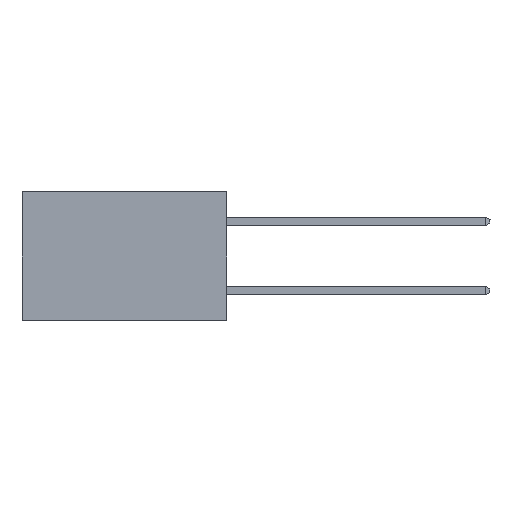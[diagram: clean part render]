
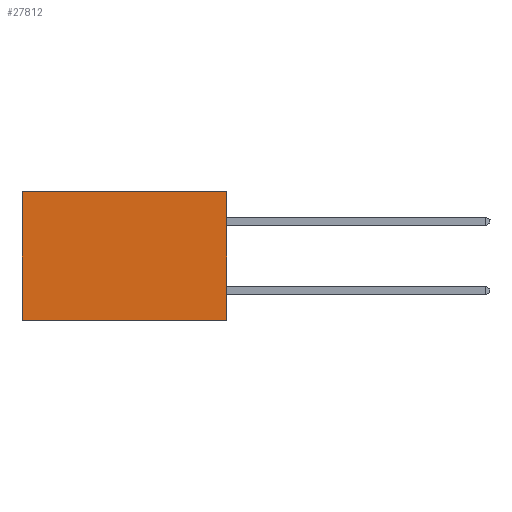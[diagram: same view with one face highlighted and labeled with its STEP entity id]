
A CAD part, left-side view. The second image highlights one B-rep face of the part: STEP entity #27812.
In plain terms, the highlighted planar face has unit normal (-1, 0, 0).
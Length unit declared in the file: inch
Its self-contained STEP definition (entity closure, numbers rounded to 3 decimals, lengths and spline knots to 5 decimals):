
#1165 = CARTESIAN_POINT ( 'NONE',  ( 0.277, 0.59, -0.37 ) ) ;
#3208 = LINE ( 'NONE', #18784, #22879 ) ;
#3996 = DIRECTION ( 'NONE',  ( 0., 0., -1. ) ) ;
#4317 = VECTOR ( 'NONE', #29599, 39.37008 ) ;
#4749 = LINE ( 'NONE', #11071, #30061 ) ;
#8733 = ORIENTED_EDGE ( 'NONE', *, *, #12134, .F. ) ;
#9128 = VERTEX_POINT ( 'NONE', #13149 ) ;
#10547 = VERTEX_POINT ( 'NONE', #1165 ) ;
#11071 = CARTESIAN_POINT ( 'NONE',  ( 0.277, 0., 0. ) ) ;
#12134 = EDGE_CURVE ( 'NONE', #9128, #20420, #3208, .T. ) ;
#12529 = CARTESIAN_POINT ( 'NONE',  ( 0.277, 0.59, -0.37 ) ) ;
#13149 = CARTESIAN_POINT ( 'NONE',  ( 0.277, 0., 0. ) ) ;
#13502 = DIRECTION ( 'NONE',  ( 0., 1., 0. ) ) ;
#13918 = EDGE_CURVE ( 'NONE', #24196, #10547, #23184, .T. ) ;
#14272 = PLANE ( 'NONE',  #29160 ) ;
#14430 = ORIENTED_EDGE ( 'NONE', *, *, #13918, .T. ) ;
#15131 = EDGE_LOOP ( 'NONE', ( #14430, #27126, #8733, #29062 ) ) ;
#16356 = CARTESIAN_POINT ( 'NONE',  ( 0.277, 0.59, 0. ) ) ;
#16778 = DIRECTION ( 'NONE',  ( 0., 0., -1. ) ) ;
#18784 = CARTESIAN_POINT ( 'NONE',  ( 0.277, 0., -0.37 ) ) ;
#20420 = VERTEX_POINT ( 'NONE', #28505 ) ;
#21054 = EDGE_CURVE ( 'NONE', #9128, #24196, #4749, .T. ) ;
#21585 = CARTESIAN_POINT ( 'NONE',  ( 0.277, 0., -0.37 ) ) ;
#22879 = VECTOR ( 'NONE', #3996, 39.37008 ) ;
#23043 = VECTOR ( 'NONE', #28591, 39.37008 ) ;
#23184 = LINE ( 'NONE', #12529, #4317 ) ;
#23723 = CARTESIAN_POINT ( 'NONE',  ( 0.277, 0., -0.37 ) ) ;
#24196 = VERTEX_POINT ( 'NONE', #16356 ) ;
#27126 = ORIENTED_EDGE ( 'NONE', *, *, #28648, .F. ) ;
#27256 = FACE_OUTER_BOUND ( 'NONE', #15131, .T. ) ;
#27812 = ADVANCED_FACE ( 'NONE', ( #27256 ), #14272, .F. ) ;
#28505 = CARTESIAN_POINT ( 'NONE',  ( 0.277, 0., -0.37 ) ) ;
#28591 = DIRECTION ( 'NONE',  ( 0., 1., 0. ) ) ;
#28648 = EDGE_CURVE ( 'NONE', #20420, #10547, #29475, .T. ) ;
#29062 = ORIENTED_EDGE ( 'NONE', *, *, #21054, .T. ) ;
#29160 = AXIS2_PLACEMENT_3D ( 'NONE', #21585, #31338, #16778 ) ;
#29475 = LINE ( 'NONE', #23723, #23043 ) ;
#29599 = DIRECTION ( 'NONE',  ( 0., 0., -1. ) ) ;
#30061 = VECTOR ( 'NONE', #13502, 39.37008 ) ;
#31338 = DIRECTION ( 'NONE',  ( 1., 0., 0. ) ) ;
